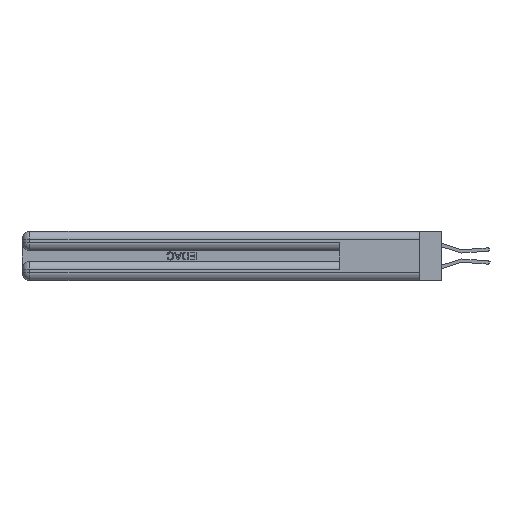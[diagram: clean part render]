
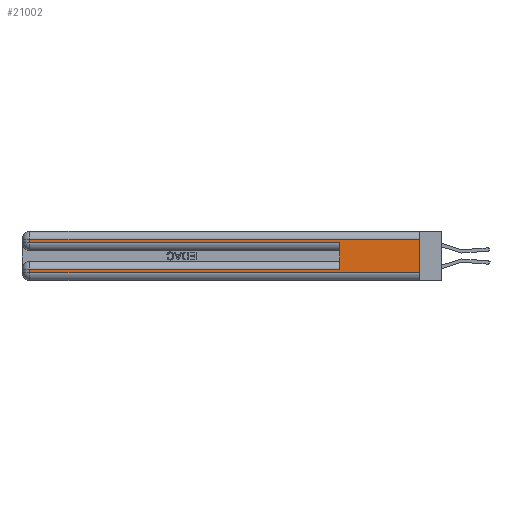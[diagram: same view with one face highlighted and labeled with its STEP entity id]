
A CAD part, left-side view. The second image highlights one B-rep face of the part: STEP entity #21002.
In plain terms, the highlighted planar face has unit normal (-1, 0, 0).
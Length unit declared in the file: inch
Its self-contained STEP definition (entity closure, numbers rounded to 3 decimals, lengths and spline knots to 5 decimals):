
#18 = EDGE_LOOP ( 'NONE', ( #1095, #29229, #27649, #29300, #30292, #44618, #32877, #13077 ) ) ;
#970 = VERTEX_POINT ( 'NONE', #11736 ) ;
#1095 = ORIENTED_EDGE ( 'NONE', *, *, #25658, .F. ) ;
#3746 = FACE_OUTER_BOUND ( 'NONE', #18, .T. ) ;
#5690 = CARTESIAN_POINT ( 'NONE',  ( 0., 2.94, 0.06 ) ) ;
#6178 = AXIS2_PLACEMENT_3D ( 'NONE', #49202, #6224, #33623 ) ;
#6192 = VERTEX_POINT ( 'NONE', #37621 ) ;
#6224 = DIRECTION ( 'NONE',  ( 1., 0., 0. ) ) ;
#6748 = CARTESIAN_POINT ( 'NONE',  ( 0., 2.94, 0.37 ) ) ;
#9011 = VECTOR ( 'NONE', #45798, 39.37008 ) ;
#9664 = CARTESIAN_POINT ( 'NONE',  ( 0., 0., 0.31 ) ) ;
#11011 = VECTOR ( 'NONE', #25749, 39.37008 ) ;
#11736 = CARTESIAN_POINT ( 'NONE',  ( 0., 2.94, 0.085 ) ) ;
#13077 = ORIENTED_EDGE ( 'NONE', *, *, #30859, .T. ) ;
#13368 = CARTESIAN_POINT ( 'NONE',  ( 0., 2.94, 0.285 ) ) ;
#14153 = EDGE_CURVE ( 'NONE', #6192, #39125, #25696, .T. ) ;
#14440 = DIRECTION ( 'NONE',  ( 0., 1., 0. ) ) ;
#18240 = VECTOR ( 'NONE', #25250, 39.37008 ) ;
#19210 = EDGE_CURVE ( 'NONE', #6192, #970, #48684, .T. ) ;
#21002 = ADVANCED_FACE ( 'NONE', ( #3746 ), #41348, .F. ) ;
#21581 = DIRECTION ( 'NONE',  ( 0., -1., 0. ) ) ;
#21834 = CARTESIAN_POINT ( 'NONE',  ( 0., 0., 0.285 ) ) ;
#22575 = VERTEX_POINT ( 'NONE', #27457 ) ;
#23903 = LINE ( 'NONE', #21834, #11011 ) ;
#24487 = VECTOR ( 'NONE', #24656, 39.37008 ) ;
#24656 = DIRECTION ( 'NONE',  ( 0., 0., 1. ) ) ;
#25250 = DIRECTION ( 'NONE',  ( 0., 0., -1. ) ) ;
#25658 = EDGE_CURVE ( 'NONE', #44088, #22575, #49376, .T. ) ;
#25696 = LINE ( 'NONE', #36282, #24487 ) ;
#25720 = CARTESIAN_POINT ( 'NONE',  ( 0., 0.6, 0.285 ) ) ;
#25749 = DIRECTION ( 'NONE',  ( 0., -1., 0. ) ) ;
#27457 = CARTESIAN_POINT ( 'NONE',  ( 0., 0., 0.06 ) ) ;
#27649 = ORIENTED_EDGE ( 'NONE', *, *, #34733, .T. ) ;
#29229 = ORIENTED_EDGE ( 'NONE', *, *, #50002, .T. ) ;
#29300 = ORIENTED_EDGE ( 'NONE', *, *, #45976, .T. ) ;
#29406 = CARTESIAN_POINT ( 'NONE',  ( 0., 0., 0.06 ) ) ;
#29970 = CARTESIAN_POINT ( 'NONE',  ( 0., 0., 0.37 ) ) ;
#30292 = ORIENTED_EDGE ( 'NONE', *, *, #14153, .F. ) ;
#30859 = EDGE_CURVE ( 'NONE', #46684, #22575, #38837, .T. ) ;
#31244 = VECTOR ( 'NONE', #44919, 39.37008 ) ;
#32877 = ORIENTED_EDGE ( 'NONE', *, *, #40936, .T. ) ;
#33623 = DIRECTION ( 'NONE',  ( 0., 0., -1. ) ) ;
#34595 = VECTOR ( 'NONE', #14440, 39.37008 ) ;
#34733 = EDGE_CURVE ( 'NONE', #48354, #41579, #41485, .T. ) ;
#36282 = CARTESIAN_POINT ( 'NONE',  ( 0., 0.6, 0.145 ) ) ;
#37601 = VECTOR ( 'NONE', #21581, 39.37008 ) ;
#37621 = CARTESIAN_POINT ( 'NONE',  ( 0., 0.6, 0.085 ) ) ;
#37760 = VECTOR ( 'NONE', #49485, 39.37008 ) ;
#38837 = LINE ( 'NONE', #29406, #37601 ) ;
#39125 = VERTEX_POINT ( 'NONE', #25720 ) ;
#40280 = LINE ( 'NONE', #48667, #18240 ) ;
#40936 = EDGE_CURVE ( 'NONE', #970, #46684, #40280, .T. ) ;
#41348 = PLANE ( 'NONE',  #6178 ) ;
#41485 = LINE ( 'NONE', #6748, #9011 ) ;
#41579 = VERTEX_POINT ( 'NONE', #13368 ) ;
#41682 = LINE ( 'NONE', #9664, #31244 ) ;
#44088 = VERTEX_POINT ( 'NONE', #46286 ) ;
#44618 = ORIENTED_EDGE ( 'NONE', *, *, #19210, .T. ) ;
#44919 = DIRECTION ( 'NONE',  ( 0., 1., 0. ) ) ;
#45764 = CARTESIAN_POINT ( 'NONE',  ( 0., 0., 0.085 ) ) ;
#45798 = DIRECTION ( 'NONE',  ( 0., 0., -1. ) ) ;
#45976 = EDGE_CURVE ( 'NONE', #41579, #39125, #23903, .T. ) ;
#46286 = CARTESIAN_POINT ( 'NONE',  ( 0., 0., 0.31 ) ) ;
#46684 = VERTEX_POINT ( 'NONE', #5690 ) ;
#48354 = VERTEX_POINT ( 'NONE', #50061 ) ;
#48667 = CARTESIAN_POINT ( 'NONE',  ( 0., 2.94, 0.37 ) ) ;
#48684 = LINE ( 'NONE', #45764, #34595 ) ;
#49202 = CARTESIAN_POINT ( 'NONE',  ( 0., 0., 0.37 ) ) ;
#49376 = LINE ( 'NONE', #29970, #37760 ) ;
#49485 = DIRECTION ( 'NONE',  ( 0., 0., -1. ) ) ;
#50002 = EDGE_CURVE ( 'NONE', #44088, #48354, #41682, .T. ) ;
#50061 = CARTESIAN_POINT ( 'NONE',  ( 0., 2.94, 0.31 ) ) ;
